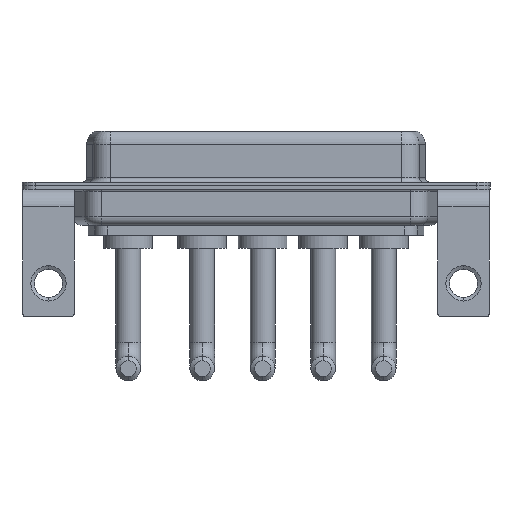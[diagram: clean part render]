
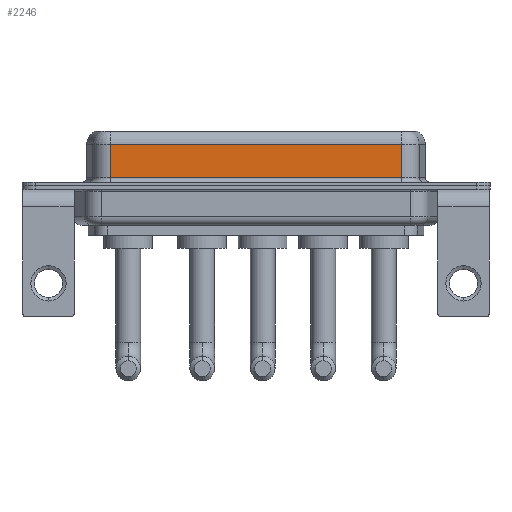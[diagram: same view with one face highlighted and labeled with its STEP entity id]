
A CAD part, front view. The second image highlights one B-rep face of the part: STEP entity #2246.
In plain terms, the highlighted planar face has unit normal (0, -1, 0).
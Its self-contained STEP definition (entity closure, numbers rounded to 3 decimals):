
#567 = ORIENTED_EDGE ( 'NONE', *, *, #13335, .T. ) ;
#871 = CARTESIAN_POINT ( 'NONE',  ( 7.013, -3.95, 4.65 ) ) ;
#1992 = DIRECTION ( 'NONE',  ( 0., 0., 1. ) ) ;
#2246 = ADVANCED_FACE ( 'NONE', ( #10275 ), #7102, .F. ) ;
#2781 = EDGE_LOOP ( 'NONE', ( #5984, #6681, #567, #11709 ) ) ;
#3452 = VECTOR ( 'NONE', #4798, 1000. ) ;
#3577 = VERTEX_POINT ( 'NONE', #6627 ) ;
#3586 = LINE ( 'NONE', #6658, #3779 ) ;
#3723 = EDGE_CURVE ( 'NONE', #10515, #13283, #7944, .T. ) ;
#3724 = CARTESIAN_POINT ( 'NONE',  ( 40.037, -3.95, 4.65 ) ) ;
#3758 = EDGE_CURVE ( 'NONE', #10515, #3849, #3827, .T. ) ;
#3779 = VECTOR ( 'NONE', #12878, 1000. ) ;
#3827 = LINE ( 'NONE', #12238, #7602 ) ;
#3849 = VERTEX_POINT ( 'NONE', #4939 ) ;
#4110 = CARTESIAN_POINT ( 'NONE',  ( 40.037, -3.95, 6.4 ) ) ;
#4798 = DIRECTION ( 'NONE',  ( -1., 0., 0. ) ) ;
#4930 = EDGE_CURVE ( 'NONE', #3577, #3849, #3586, .T. ) ;
#4939 = CARTESIAN_POINT ( 'NONE',  ( 40.037, -3.95, 0.9 ) ) ;
#5984 = ORIENTED_EDGE ( 'NONE', *, *, #3758, .F. ) ;
#6627 = CARTESIAN_POINT ( 'NONE',  ( 7.013, -3.95, 0.9 ) ) ;
#6658 = CARTESIAN_POINT ( 'NONE',  ( 40.037, -3.95, 0.9 ) ) ;
#6681 = ORIENTED_EDGE ( 'NONE', *, *, #3723, .T. ) ;
#6994 = VECTOR ( 'NONE', #12350, 1000. ) ;
#7087 = CARTESIAN_POINT ( 'NONE',  ( 7.013, -3.95, 6.4 ) ) ;
#7102 = PLANE ( 'NONE',  #9105 ) ;
#7313 = DIRECTION ( 'NONE',  ( 0., 1., 0. ) ) ;
#7602 = VECTOR ( 'NONE', #8080, 1000. ) ;
#7944 = LINE ( 'NONE', #11283, #3452 ) ;
#8080 = DIRECTION ( 'NONE',  ( 0., 0., -1. ) ) ;
#9105 = AXIS2_PLACEMENT_3D ( 'NONE', #4110, #7313, #1992 ) ;
#10275 = FACE_OUTER_BOUND ( 'NONE', #2781, .T. ) ;
#10515 = VERTEX_POINT ( 'NONE', #3724 ) ;
#11283 = CARTESIAN_POINT ( 'NONE',  ( 40.037, -3.95, 4.65 ) ) ;
#11709 = ORIENTED_EDGE ( 'NONE', *, *, #4930, .T. ) ;
#12238 = CARTESIAN_POINT ( 'NONE',  ( 40.037, -3.95, 6.4 ) ) ;
#12286 = LINE ( 'NONE', #7087, #6994 ) ;
#12350 = DIRECTION ( 'NONE',  ( 0., 0., -1. ) ) ;
#12878 = DIRECTION ( 'NONE',  ( 1., 0., 0. ) ) ;
#13283 = VERTEX_POINT ( 'NONE', #871 ) ;
#13335 = EDGE_CURVE ( 'NONE', #13283, #3577, #12286, .T. ) ;
